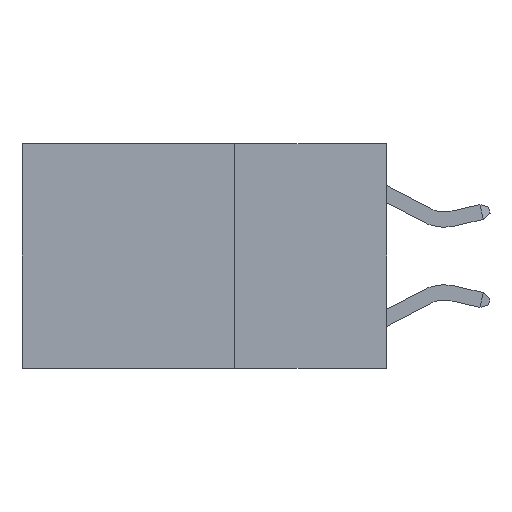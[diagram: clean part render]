
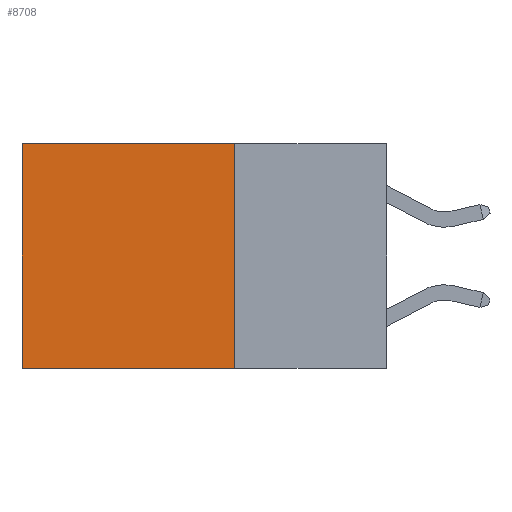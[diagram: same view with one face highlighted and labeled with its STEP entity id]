
A CAD part, left-side view. The second image highlights one B-rep face of the part: STEP entity #8708.
In plain terms, the highlighted planar face has unit normal (-1, 0, 0).
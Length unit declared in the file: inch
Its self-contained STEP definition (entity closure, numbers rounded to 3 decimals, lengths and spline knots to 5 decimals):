
#27 = CARTESIAN_POINT ( 'NONE',  ( 0.2625, 0.6, -0.37 ) ) ;
#1466 = CARTESIAN_POINT ( 'NONE',  ( 0.2625, 0.6, 0. ) ) ;
#2589 = VERTEX_POINT ( 'NONE', #27 ) ;
#2644 = ORIENTED_EDGE ( 'NONE', *, *, #18246, .F. ) ;
#2721 = FACE_OUTER_BOUND ( 'NONE', #11486, .T. ) ;
#3302 = PLANE ( 'NONE',  #20153 ) ;
#3483 = CARTESIAN_POINT ( 'NONE',  ( 0.2625, 0.25, 0. ) ) ;
#5494 = EDGE_CURVE ( 'NONE', #8263, #2589, #10014, .T. ) ;
#5623 = CARTESIAN_POINT ( 'NONE',  ( 0.2625, 0.25, -0.37 ) ) ;
#6079 = EDGE_CURVE ( 'NONE', #18384, #2589, #8366, .T. ) ;
#8263 = VERTEX_POINT ( 'NONE', #5623 ) ;
#8366 = LINE ( 'NONE', #1466, #27781 ) ;
#8708 = ADVANCED_FACE ( 'NONE', ( #2721 ), #3302, .F. ) ;
#9171 = CARTESIAN_POINT ( 'NONE',  ( 0.2625, 0.25, 0. ) ) ;
#9727 = DIRECTION ( 'NONE',  ( 0., 1., 0. ) ) ;
#9850 = DIRECTION ( 'NONE',  ( 0., 0., -1. ) ) ;
#10014 = LINE ( 'NONE', #24893, #19227 ) ;
#10311 = VECTOR ( 'NONE', #12255, 39.37008 ) ;
#11486 = EDGE_LOOP ( 'NONE', ( #23672, #27533, #2644, #16032 ) ) ;
#11624 = CARTESIAN_POINT ( 'NONE',  ( 0.2625, 0.25, 0. ) ) ;
#12063 = DIRECTION ( 'NONE',  ( 1., 0., 0. ) ) ;
#12255 = DIRECTION ( 'NONE',  ( 0., 1., 0. ) ) ;
#14255 = EDGE_CURVE ( 'NONE', #17586, #18384, #25412, .T. ) ;
#16032 = ORIENTED_EDGE ( 'NONE', *, *, #14255, .T. ) ;
#17256 = CARTESIAN_POINT ( 'NONE',  ( 0.2625, 0.6, 0. ) ) ;
#17586 = VERTEX_POINT ( 'NONE', #9171 ) ;
#18166 = CARTESIAN_POINT ( 'NONE',  ( 0.2625, 0.25, 0. ) ) ;
#18246 = EDGE_CURVE ( 'NONE', #17586, #8263, #25691, .T. ) ;
#18384 = VERTEX_POINT ( 'NONE', #17256 ) ;
#19227 = VECTOR ( 'NONE', #9727, 39.37008 ) ;
#20153 = AXIS2_PLACEMENT_3D ( 'NONE', #11624, #12063, #26813 ) ;
#23672 = ORIENTED_EDGE ( 'NONE', *, *, #6079, .T. ) ;
#24893 = CARTESIAN_POINT ( 'NONE',  ( 0.2625, 0.25, -0.37 ) ) ;
#25279 = DIRECTION ( 'NONE',  ( 0., 0., -1. ) ) ;
#25412 = LINE ( 'NONE', #3483, #10311 ) ;
#25691 = LINE ( 'NONE', #18166, #25916 ) ;
#25916 = VECTOR ( 'NONE', #9850, 39.37008 ) ;
#26813 = DIRECTION ( 'NONE',  ( 0., 0., -1. ) ) ;
#27533 = ORIENTED_EDGE ( 'NONE', *, *, #5494, .F. ) ;
#27781 = VECTOR ( 'NONE', #25279, 39.37008 ) ;
